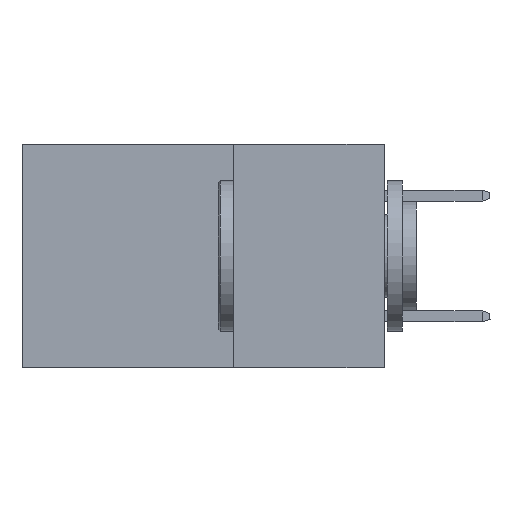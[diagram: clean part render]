
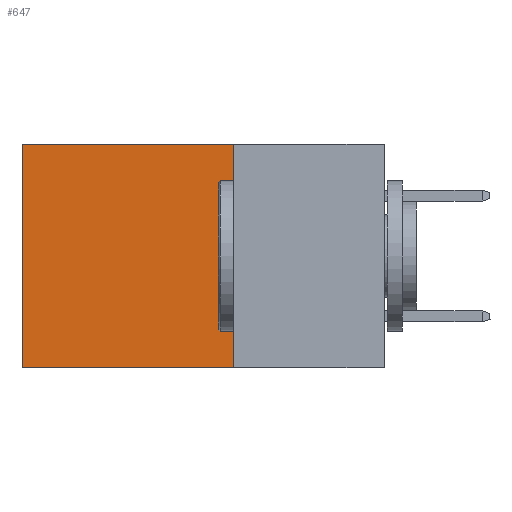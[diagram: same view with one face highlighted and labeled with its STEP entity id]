
A CAD part, left-side view. The second image highlights one B-rep face of the part: STEP entity #647.
In plain terms, the highlighted planar face has unit normal (-1, 0, 0).
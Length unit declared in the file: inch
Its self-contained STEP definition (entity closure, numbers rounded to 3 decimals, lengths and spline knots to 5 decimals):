
#220 = ORIENTED_EDGE ( 'NONE', *, *, #11065, .F. ) ;
#299 = CARTESIAN_POINT ( 'NONE',  ( 0.2615, 0.25, -0.37 ) ) ;
#321 = AXIS2_PLACEMENT_3D ( 'NONE', #858, #15946, #16214 ) ;
#647 = ADVANCED_FACE ( 'NONE', ( #8040 ), #12246, .F. ) ;
#858 = CARTESIAN_POINT ( 'NONE',  ( 0.2615, 0.25, -0.37 ) ) ;
#1239 = CARTESIAN_POINT ( 'NONE',  ( 0.2615, 0.6, 0. ) ) ;
#1857 = VECTOR ( 'NONE', #5289, 39.37008 ) ;
#1910 = DIRECTION ( 'NONE',  ( 0., 0., -1. ) ) ;
#2349 = CARTESIAN_POINT ( 'NONE',  ( 0.2615, 0.25, -0.37 ) ) ;
#2819 = EDGE_CURVE ( 'NONE', #19578, #15779, #6563, .T. ) ;
#3430 = EDGE_LOOP ( 'NONE', ( #12004, #220, #12338, #6912 ) ) ;
#3436 = EDGE_CURVE ( 'NONE', #19578, #7458, #14189, .T. ) ;
#3626 = DIRECTION ( 'NONE',  ( 0., 0., -1. ) ) ;
#5289 = DIRECTION ( 'NONE',  ( 0., 1., 0. ) ) ;
#6563 = LINE ( 'NONE', #8296, #1857 ) ;
#6912 = ORIENTED_EDGE ( 'NONE', *, *, #2819, .T. ) ;
#7458 = VERTEX_POINT ( 'NONE', #299 ) ;
#8040 = FACE_OUTER_BOUND ( 'NONE', #3430, .T. ) ;
#8296 = CARTESIAN_POINT ( 'NONE',  ( 0.2615, 0.25, 0. ) ) ;
#8477 = VECTOR ( 'NONE', #17603, 39.37008 ) ;
#8854 = CARTESIAN_POINT ( 'NONE',  ( 0.2615, 0.6, -0.37 ) ) ;
#11065 = EDGE_CURVE ( 'NONE', #7458, #21234, #17714, .T. ) ;
#12004 = ORIENTED_EDGE ( 'NONE', *, *, #21958, .T. ) ;
#12009 = VECTOR ( 'NONE', #3626, 39.37008 ) ;
#12246 = PLANE ( 'NONE',  #321 ) ;
#12338 = ORIENTED_EDGE ( 'NONE', *, *, #3436, .F. ) ;
#14189 = LINE ( 'NONE', #2349, #17140 ) ;
#15394 = CARTESIAN_POINT ( 'NONE',  ( 0.2615, 0.6, -0.37 ) ) ;
#15779 = VERTEX_POINT ( 'NONE', #1239 ) ;
#15946 = DIRECTION ( 'NONE',  ( 1., 0., 0. ) ) ;
#16214 = DIRECTION ( 'NONE',  ( 0., 0., -1. ) ) ;
#16592 = LINE ( 'NONE', #8854, #12009 ) ;
#17140 = VECTOR ( 'NONE', #1910, 39.37008 ) ;
#17603 = DIRECTION ( 'NONE',  ( 0., 1., 0. ) ) ;
#17714 = LINE ( 'NONE', #21012, #8477 ) ;
#19578 = VERTEX_POINT ( 'NONE', #21071 ) ;
#21012 = CARTESIAN_POINT ( 'NONE',  ( 0.2615, 0.25, -0.37 ) ) ;
#21071 = CARTESIAN_POINT ( 'NONE',  ( 0.2615, 0.25, 0. ) ) ;
#21234 = VERTEX_POINT ( 'NONE', #15394 ) ;
#21958 = EDGE_CURVE ( 'NONE', #15779, #21234, #16592, .T. ) ;
